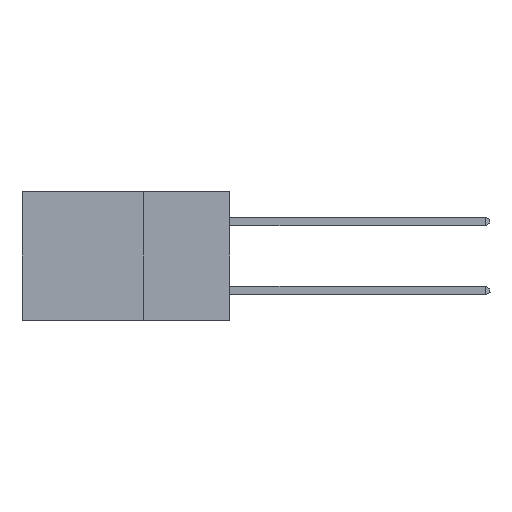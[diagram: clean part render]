
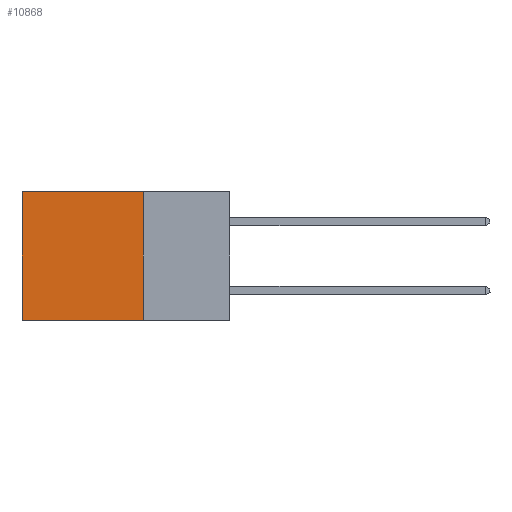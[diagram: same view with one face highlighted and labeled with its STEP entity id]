
A CAD part, left-side view. The second image highlights one B-rep face of the part: STEP entity #10868.
In plain terms, the highlighted planar face has unit normal (-1, 0, 0).
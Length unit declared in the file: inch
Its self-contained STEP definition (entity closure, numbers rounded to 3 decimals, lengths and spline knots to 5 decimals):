
#255 = CARTESIAN_POINT ( 'NONE',  ( 0.298, 0.6, -0.37 ) ) ;
#512 = VERTEX_POINT ( 'NONE', #566 ) ;
#566 = CARTESIAN_POINT ( 'NONE',  ( 0.298, 0.25, 0. ) ) ;
#1394 = AXIS2_PLACEMENT_3D ( 'NONE', #10844, #3874, #13726 ) ;
#1549 = DIRECTION ( 'NONE',  ( 0., 0., -1. ) ) ;
#1602 = DIRECTION ( 'NONE',  ( 0., 1., 0. ) ) ;
#2322 = ORIENTED_EDGE ( 'NONE', *, *, #15517, .F. ) ;
#3351 = VECTOR ( 'NONE', #1549, 39.37008 ) ;
#3538 = LINE ( 'NONE', #7000, #11454 ) ;
#3874 = DIRECTION ( 'NONE',  ( 1., 0., 0. ) ) ;
#4169 = CARTESIAN_POINT ( 'NONE',  ( 0.298, 0.6, 0. ) ) ;
#4543 = CARTESIAN_POINT ( 'NONE',  ( 0.298, 0.25, -0.37 ) ) ;
#4869 = DIRECTION ( 'NONE',  ( 0., 0., -1. ) ) ;
#6444 = VECTOR ( 'NONE', #8722, 39.37008 ) ;
#6958 = VERTEX_POINT ( 'NONE', #4169 ) ;
#7000 = CARTESIAN_POINT ( 'NONE',  ( 0.298, 0.25, 0. ) ) ;
#7419 = CARTESIAN_POINT ( 'NONE',  ( 0.298, 0.25, -0.37 ) ) ;
#8403 = LINE ( 'NONE', #4543, #6444 ) ;
#8722 = DIRECTION ( 'NONE',  ( 0., 1., 0. ) ) ;
#9418 = PLANE ( 'NONE',  #1394 ) ;
#9490 = LINE ( 'NONE', #11311, #3351 ) ;
#9599 = EDGE_CURVE ( 'NONE', #512, #6958, #3538, .T. ) ;
#10155 = VECTOR ( 'NONE', #4869, 39.37008 ) ;
#10688 = EDGE_LOOP ( 'NONE', ( #16132, #13284, #2322, #14098 ) ) ;
#10844 = CARTESIAN_POINT ( 'NONE',  ( 0.298, 0.25, 0. ) ) ;
#10868 = ADVANCED_FACE ( 'NONE', ( #17588 ), #9418, .F. ) ;
#11311 = CARTESIAN_POINT ( 'NONE',  ( 0.298, 0.6, 0. ) ) ;
#11454 = VECTOR ( 'NONE', #1602, 39.37008 ) ;
#12283 = VERTEX_POINT ( 'NONE', #7419 ) ;
#13284 = ORIENTED_EDGE ( 'NONE', *, *, #14179, .F. ) ;
#13726 = DIRECTION ( 'NONE',  ( 0., 0., -1. ) ) ;
#14098 = ORIENTED_EDGE ( 'NONE', *, *, #9599, .T. ) ;
#14179 = EDGE_CURVE ( 'NONE', #12283, #16391, #8403, .T. ) ;
#15517 = EDGE_CURVE ( 'NONE', #512, #12283, #16301, .T. ) ;
#15931 = EDGE_CURVE ( 'NONE', #6958, #16391, #9490, .T. ) ;
#16132 = ORIENTED_EDGE ( 'NONE', *, *, #15931, .T. ) ;
#16301 = LINE ( 'NONE', #17549, #10155 ) ;
#16391 = VERTEX_POINT ( 'NONE', #255 ) ;
#17549 = CARTESIAN_POINT ( 'NONE',  ( 0.298, 0.25, 0. ) ) ;
#17588 = FACE_OUTER_BOUND ( 'NONE', #10688, .T. ) ;
